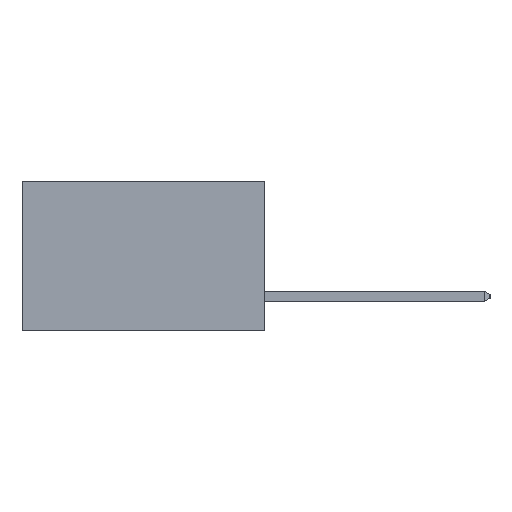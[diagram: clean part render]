
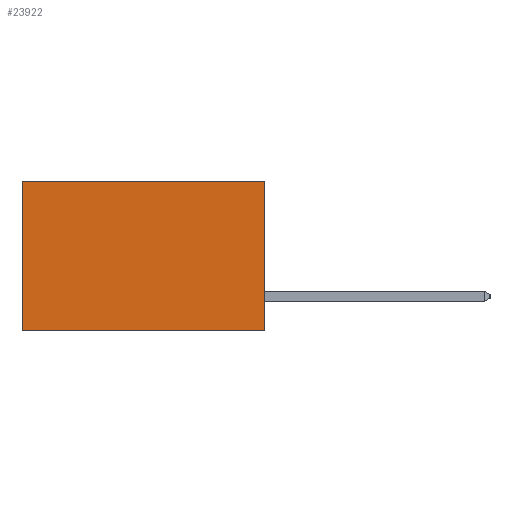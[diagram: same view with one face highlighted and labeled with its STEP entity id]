
A CAD part, left-side view. The second image highlights one B-rep face of the part: STEP entity #23922.
In plain terms, the highlighted planar face has unit normal (-1, 0, 0).
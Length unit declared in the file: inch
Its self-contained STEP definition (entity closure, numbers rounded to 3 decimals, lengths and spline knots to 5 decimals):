
#1352 = VECTOR ( 'NONE', #17579, 39.37008 ) ;
#2188 = DIRECTION ( 'NONE',  ( 0., 0., -1. ) ) ;
#2608 = ORIENTED_EDGE ( 'NONE', *, *, #4053, .F. ) ;
#2978 = VECTOR ( 'NONE', #22713, 39.37008 ) ;
#4053 = EDGE_CURVE ( 'NONE', #5982, #15846, #13000, .T. ) ;
#4132 = LINE ( 'NONE', #5393, #9159 ) ;
#5393 = CARTESIAN_POINT ( 'NONE',  ( 0.2615, 0., 0. ) ) ;
#5982 = VERTEX_POINT ( 'NONE', #21032 ) ;
#7536 = AXIS2_PLACEMENT_3D ( 'NONE', #22016, #11116, #23789 ) ;
#8014 = EDGE_LOOP ( 'NONE', ( #21450, #2608, #12644, #13323 ) ) ;
#8165 = FACE_OUTER_BOUND ( 'NONE', #8014, .T. ) ;
#9159 = VECTOR ( 'NONE', #11029, 39.37008 ) ;
#11029 = DIRECTION ( 'NONE',  ( 0., 1., 0. ) ) ;
#11066 = CARTESIAN_POINT ( 'NONE',  ( 0.2615, 0.6, 0. ) ) ;
#11116 = DIRECTION ( 'NONE',  ( 1., 0., 0. ) ) ;
#12644 = ORIENTED_EDGE ( 'NONE', *, *, #23591, .F. ) ;
#13000 = LINE ( 'NONE', #22696, #2978 ) ;
#13323 = ORIENTED_EDGE ( 'NONE', *, *, #22067, .T. ) ;
#13831 = LINE ( 'NONE', #17212, #22854 ) ;
#13898 = CARTESIAN_POINT ( 'NONE',  ( 0.2615, 0.6, -0.37 ) ) ;
#15083 = VERTEX_POINT ( 'NONE', #17164 ) ;
#15716 = CARTESIAN_POINT ( 'NONE',  ( 0.2615, 0., -0.37 ) ) ;
#15846 = VERTEX_POINT ( 'NONE', #13898 ) ;
#16355 = LINE ( 'NONE', #15716, #1352 ) ;
#17164 = CARTESIAN_POINT ( 'NONE',  ( 0.2615, 0., 0. ) ) ;
#17212 = CARTESIAN_POINT ( 'NONE',  ( 0.2615, 0.6, -0.37 ) ) ;
#17277 = VERTEX_POINT ( 'NONE', #11066 ) ;
#17579 = DIRECTION ( 'NONE',  ( 0., 0., -1. ) ) ;
#18479 = PLANE ( 'NONE',  #7536 ) ;
#21032 = CARTESIAN_POINT ( 'NONE',  ( 0.2615, 0., -0.37 ) ) ;
#21450 = ORIENTED_EDGE ( 'NONE', *, *, #22279, .T. ) ;
#22016 = CARTESIAN_POINT ( 'NONE',  ( 0.2615, 0., -0.37 ) ) ;
#22067 = EDGE_CURVE ( 'NONE', #15083, #17277, #4132, .T. ) ;
#22279 = EDGE_CURVE ( 'NONE', #17277, #15846, #13831, .T. ) ;
#22696 = CARTESIAN_POINT ( 'NONE',  ( 0.2615, 0., -0.37 ) ) ;
#22713 = DIRECTION ( 'NONE',  ( 0., 1., 0. ) ) ;
#22854 = VECTOR ( 'NONE', #2188, 39.37008 ) ;
#23591 = EDGE_CURVE ( 'NONE', #15083, #5982, #16355, .T. ) ;
#23789 = DIRECTION ( 'NONE',  ( 0., 0., -1. ) ) ;
#23922 = ADVANCED_FACE ( 'NONE', ( #8165 ), #18479, .F. ) ;
